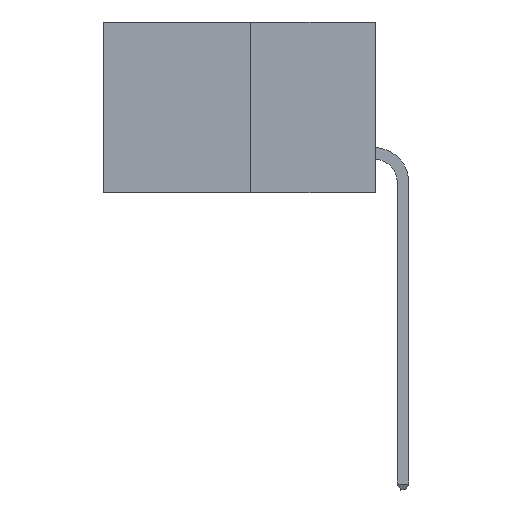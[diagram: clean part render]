
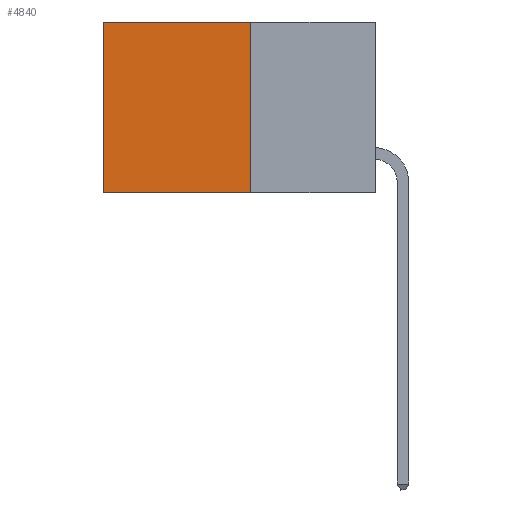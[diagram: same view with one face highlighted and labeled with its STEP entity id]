
A CAD part, left-side view. The second image highlights one B-rep face of the part: STEP entity #4840.
In plain terms, the highlighted planar face has unit normal (-1, 0, 0).
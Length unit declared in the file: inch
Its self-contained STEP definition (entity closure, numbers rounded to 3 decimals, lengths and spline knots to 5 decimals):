
#4840 = ADVANCED_FACE ( 'NONE', ( #11336 ), #29090, .F. ) ;
#5034 = LINE ( 'NONE', #22589, #17401 ) ;
#5038 = ORIENTED_EDGE ( 'NONE', *, *, #12102, .F. ) ;
#8185 = CARTESIAN_POINT ( 'NONE',  ( 0.277, 0.59, -0.37 ) ) ;
#8556 = VERTEX_POINT ( 'NONE', #24709 ) ;
#11336 = FACE_OUTER_BOUND ( 'NONE', #11481, .T. ) ;
#11481 = EDGE_LOOP ( 'NONE', ( #12978, #5038, #29026, #19945 ) ) ;
#12102 = EDGE_CURVE ( 'NONE', #8556, #26108, #5034, .T. ) ;
#12290 = EDGE_CURVE ( 'NONE', #18816, #8556, #29761, .T. ) ;
#12432 = VERTEX_POINT ( 'NONE', #17790 ) ;
#12978 = ORIENTED_EDGE ( 'NONE', *, *, #19864, .T. ) ;
#14653 = EDGE_CURVE ( 'NONE', #18816, #12432, #19435, .T. ) ;
#14907 = AXIS2_PLACEMENT_3D ( 'NONE', #30440, #30402, #30535 ) ;
#15243 = CARTESIAN_POINT ( 'NONE',  ( 0.277, 0.59, -0.37 ) ) ;
#16428 = LINE ( 'NONE', #15243, #22122 ) ;
#16991 = VECTOR ( 'NONE', #19615, 39.37008 ) ;
#17401 = VECTOR ( 'NONE', #22680, 39.37008 ) ;
#17684 = DIRECTION ( 'NONE',  ( 0., 0., -1. ) ) ;
#17790 = CARTESIAN_POINT ( 'NONE',  ( 0.277, 0.59, 0. ) ) ;
#18816 = VERTEX_POINT ( 'NONE', #19642 ) ;
#19435 = LINE ( 'NONE', #25642, #31340 ) ;
#19615 = DIRECTION ( 'NONE',  ( 0., 0., -1. ) ) ;
#19642 = CARTESIAN_POINT ( 'NONE',  ( 0.277, 0.27, 0. ) ) ;
#19818 = CARTESIAN_POINT ( 'NONE',  ( 0.277, 0.27, -0.37 ) ) ;
#19864 = EDGE_CURVE ( 'NONE', #12432, #26108, #16428, .T. ) ;
#19945 = ORIENTED_EDGE ( 'NONE', *, *, #14653, .T. ) ;
#22122 = VECTOR ( 'NONE', #17684, 39.37008 ) ;
#22589 = CARTESIAN_POINT ( 'NONE',  ( 0.277, 0.27, -0.37 ) ) ;
#22680 = DIRECTION ( 'NONE',  ( 0., 1., 0. ) ) ;
#24709 = CARTESIAN_POINT ( 'NONE',  ( 0.277, 0.27, -0.37 ) ) ;
#25642 = CARTESIAN_POINT ( 'NONE',  ( 0.277, 0.27, 0. ) ) ;
#26108 = VERTEX_POINT ( 'NONE', #8185 ) ;
#28046 = DIRECTION ( 'NONE',  ( 0., 1., 0. ) ) ;
#29026 = ORIENTED_EDGE ( 'NONE', *, *, #12290, .F. ) ;
#29090 = PLANE ( 'NONE',  #14907 ) ;
#29761 = LINE ( 'NONE', #19818, #16991 ) ;
#30402 = DIRECTION ( 'NONE',  ( 1., 0., 0. ) ) ;
#30440 = CARTESIAN_POINT ( 'NONE',  ( 0.277, 0.27, -0.37 ) ) ;
#30535 = DIRECTION ( 'NONE',  ( 0., 0., -1. ) ) ;
#31340 = VECTOR ( 'NONE', #28046, 39.37008 ) ;
